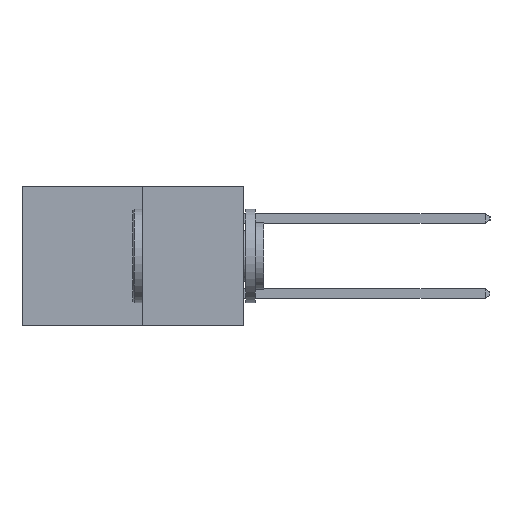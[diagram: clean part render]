
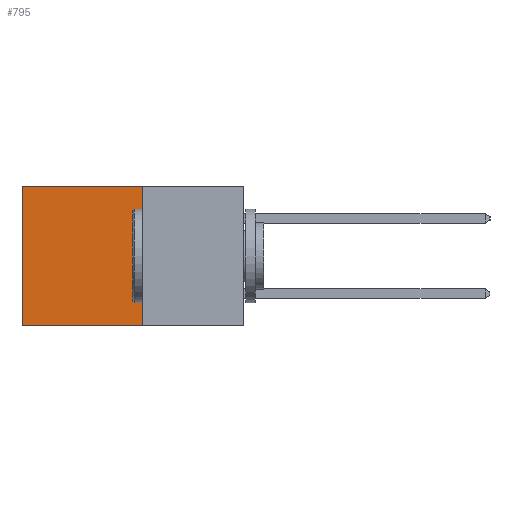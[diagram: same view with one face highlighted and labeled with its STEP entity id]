
A CAD part, left-side view. The second image highlights one B-rep face of the part: STEP entity #795.
In plain terms, the highlighted planar face has unit normal (-1, 0, 0).
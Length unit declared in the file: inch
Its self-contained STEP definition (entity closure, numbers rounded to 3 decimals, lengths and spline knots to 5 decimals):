
#49 = VECTOR ( 'NONE', #12648, 39.37008 ) ;
#203 = ORIENTED_EDGE ( 'NONE', *, *, #7049, .T. ) ;
#271 = CARTESIAN_POINT ( 'NONE',  ( 0.277, 0.59, 0. ) ) ;
#793 = LINE ( 'NONE', #7392, #13098 ) ;
#795 = ADVANCED_FACE ( 'NONE', ( #7515 ), #4598, .F. ) ;
#2980 = VERTEX_POINT ( 'NONE', #271 ) ;
#3613 = DIRECTION ( 'NONE',  ( 1., 0., 0. ) ) ;
#4375 = CARTESIAN_POINT ( 'NONE',  ( 0.277, 0.59, -0.37 ) ) ;
#4508 = DIRECTION ( 'NONE',  ( 0., 0., -1. ) ) ;
#4598 = PLANE ( 'NONE',  #7821 ) ;
#4669 = VERTEX_POINT ( 'NONE', #5818 ) ;
#4751 = ORIENTED_EDGE ( 'NONE', *, *, #5851, .T. ) ;
#4972 = EDGE_CURVE ( 'NONE', #4669, #6311, #6115, .T. ) ;
#5818 = CARTESIAN_POINT ( 'NONE',  ( 0.277, 0.27, 0. ) ) ;
#5851 = EDGE_CURVE ( 'NONE', #4669, #2980, #7222, .T. ) ;
#6095 = EDGE_CURVE ( 'NONE', #6311, #9008, #793, .T. ) ;
#6115 = LINE ( 'NONE', #11820, #12061 ) ;
#6311 = VERTEX_POINT ( 'NONE', #11429 ) ;
#6392 = CARTESIAN_POINT ( 'NONE',  ( 0.277, 0.27, -0.37 ) ) ;
#6425 = VECTOR ( 'NONE', #7301, 39.37008 ) ;
#6792 = LINE ( 'NONE', #7503, #6425 ) ;
#6974 = ORIENTED_EDGE ( 'NONE', *, *, #4972, .F. ) ;
#7049 = EDGE_CURVE ( 'NONE', #2980, #9008, #6792, .T. ) ;
#7222 = LINE ( 'NONE', #11545, #49 ) ;
#7301 = DIRECTION ( 'NONE',  ( 0., 0., -1. ) ) ;
#7392 = CARTESIAN_POINT ( 'NONE',  ( 0.277, 0.27, -0.37 ) ) ;
#7503 = CARTESIAN_POINT ( 'NONE',  ( 0.277, 0.59, -0.37 ) ) ;
#7515 = FACE_OUTER_BOUND ( 'NONE', #9590, .T. ) ;
#7821 = AXIS2_PLACEMENT_3D ( 'NONE', #6392, #3613, #4508 ) ;
#9008 = VERTEX_POINT ( 'NONE', #4375 ) ;
#9590 = EDGE_LOOP ( 'NONE', ( #203, #13578, #6974, #4751 ) ) ;
#11016 = DIRECTION ( 'NONE',  ( 0., 1., 0. ) ) ;
#11429 = CARTESIAN_POINT ( 'NONE',  ( 0.277, 0.27, -0.37 ) ) ;
#11545 = CARTESIAN_POINT ( 'NONE',  ( 0.277, 0.27, 0. ) ) ;
#11575 = DIRECTION ( 'NONE',  ( 0., 0., -1. ) ) ;
#11820 = CARTESIAN_POINT ( 'NONE',  ( 0.277, 0.27, -0.37 ) ) ;
#12061 = VECTOR ( 'NONE', #11575, 39.37008 ) ;
#12648 = DIRECTION ( 'NONE',  ( 0., 1., 0. ) ) ;
#13098 = VECTOR ( 'NONE', #11016, 39.37008 ) ;
#13578 = ORIENTED_EDGE ( 'NONE', *, *, #6095, .F. ) ;
